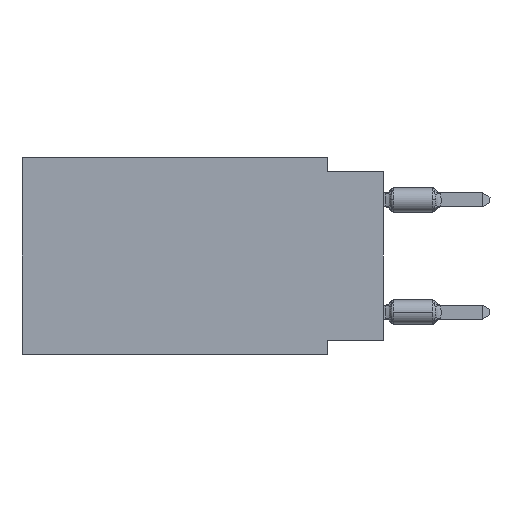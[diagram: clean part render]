
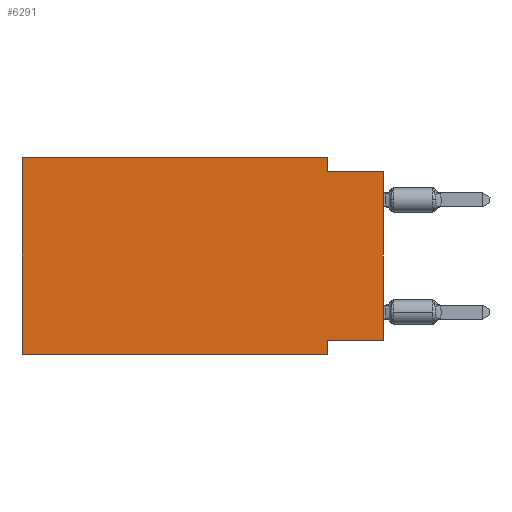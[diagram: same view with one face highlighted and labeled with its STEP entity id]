
A CAD part, left-side view. The second image highlights one B-rep face of the part: STEP entity #6291.
In plain terms, the highlighted planar face has unit normal (-1, 0, 0).
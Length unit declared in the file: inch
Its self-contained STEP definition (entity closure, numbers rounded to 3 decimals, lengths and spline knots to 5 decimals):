
#45 = LINE ( 'NONE', #5375, #10427 ) ;
#446 = CARTESIAN_POINT ( 'NONE',  ( 0., 0., -0.025 ) ) ;
#465 = VERTEX_POINT ( 'NONE', #10690 ) ;
#578 = EDGE_CURVE ( 'NONE', #5020, #465, #1015, .T. ) ;
#708 = VECTOR ( 'NONE', #12342, 39.37008 ) ;
#867 = CARTESIAN_POINT ( 'NONE',  ( 0., 0.645, 0. ) ) ;
#999 = ORIENTED_EDGE ( 'NONE', *, *, #6677, .F. ) ;
#1015 = LINE ( 'NONE', #8559, #12239 ) ;
#1303 = DIRECTION ( 'NONE',  ( 0., -1., 0. ) ) ;
#1345 = VERTEX_POINT ( 'NONE', #13321 ) ;
#1365 = VERTEX_POINT ( 'NONE', #867 ) ;
#1923 = EDGE_CURVE ( 'NONE', #1345, #16106, #2112, .T. ) ;
#1957 = LINE ( 'NONE', #7144, #708 ) ;
#2112 = LINE ( 'NONE', #8470, #4435 ) ;
#2314 = CARTESIAN_POINT ( 'NONE',  ( 0., 0.645, -0.35 ) ) ;
#3099 = VECTOR ( 'NONE', #15239, 39.37008 ) ;
#3431 = ORIENTED_EDGE ( 'NONE', *, *, #15196, .T. ) ;
#4435 = VECTOR ( 'NONE', #7371, 39.37008 ) ;
#4548 = EDGE_CURVE ( 'NONE', #10278, #1345, #4813, .T. ) ;
#4651 = CARTESIAN_POINT ( 'NONE',  ( 0., 0., -0.325 ) ) ;
#4769 = ORIENTED_EDGE ( 'NONE', *, *, #1923, .F. ) ;
#4813 = LINE ( 'NONE', #4651, #7572 ) ;
#5020 = VERTEX_POINT ( 'NONE', #15263 ) ;
#5375 = CARTESIAN_POINT ( 'NONE',  ( 0., 0.645, -0.35 ) ) ;
#5572 = DIRECTION ( 'NONE',  ( 1., 0., 0. ) ) ;
#5813 = PLANE ( 'NONE',  #16420 ) ;
#6208 = LINE ( 'NONE', #16662, #3099 ) ;
#6236 = ORIENTED_EDGE ( 'NONE', *, *, #12957, .F. ) ;
#6291 = ADVANCED_FACE ( 'NONE', ( #8270 ), #5813, .F. ) ;
#6677 = EDGE_CURVE ( 'NONE', #465, #10074, #1957, .T. ) ;
#7144 = CARTESIAN_POINT ( 'NONE',  ( 0., 0., -0.025 ) ) ;
#7352 = DIRECTION ( 'NONE',  ( 0., 1., 0. ) ) ;
#7371 = DIRECTION ( 'NONE',  ( 0., 0., -1. ) ) ;
#7572 = VECTOR ( 'NONE', #7352, 39.37008 ) ;
#7975 = ORIENTED_EDGE ( 'NONE', *, *, #4548, .F. ) ;
#8068 = EDGE_LOOP ( 'NONE', ( #3431, #999, #8498, #12904, #6236, #13268, #4769, #7975 ) ) ;
#8270 = FACE_OUTER_BOUND ( 'NONE', #8068, .T. ) ;
#8356 = DIRECTION ( 'NONE',  ( 0., 0., -1. ) ) ;
#8470 = CARTESIAN_POINT ( 'NONE',  ( 0., 0.1, -0.35 ) ) ;
#8498 = ORIENTED_EDGE ( 'NONE', *, *, #578, .F. ) ;
#8559 = CARTESIAN_POINT ( 'NONE',  ( 0., 0.1, 0. ) ) ;
#8575 = VECTOR ( 'NONE', #11095, 39.37008 ) ;
#9460 = CARTESIAN_POINT ( 'NONE',  ( 0., 0.645, 0. ) ) ;
#9985 = CARTESIAN_POINT ( 'NONE',  ( 0., 0.1, -0.35 ) ) ;
#10016 = DIRECTION ( 'NONE',  ( 0., 0., -1. ) ) ;
#10074 = VERTEX_POINT ( 'NONE', #446 ) ;
#10131 = CARTESIAN_POINT ( 'NONE',  ( 0., 0., -0.325 ) ) ;
#10278 = VERTEX_POINT ( 'NONE', #10131 ) ;
#10427 = VECTOR ( 'NONE', #1303, 39.37008 ) ;
#10690 = CARTESIAN_POINT ( 'NONE',  ( 0., 0.1, -0.025 ) ) ;
#10952 = VECTOR ( 'NONE', #15120, 39.37008 ) ;
#11095 = DIRECTION ( 'NONE',  ( 0., 0., 1. ) ) ;
#11168 = LINE ( 'NONE', #13772, #10952 ) ;
#11470 = VERTEX_POINT ( 'NONE', #2314 ) ;
#12239 = VECTOR ( 'NONE', #10016, 39.37008 ) ;
#12251 = EDGE_CURVE ( 'NONE', #1365, #5020, #11168, .T. ) ;
#12342 = DIRECTION ( 'NONE',  ( 0., -1., 0. ) ) ;
#12904 = ORIENTED_EDGE ( 'NONE', *, *, #12251, .F. ) ;
#12957 = EDGE_CURVE ( 'NONE', #11470, #1365, #6208, .T. ) ;
#13268 = ORIENTED_EDGE ( 'NONE', *, *, #16255, .T. ) ;
#13321 = CARTESIAN_POINT ( 'NONE',  ( 0., 0.1, -0.325 ) ) ;
#13772 = CARTESIAN_POINT ( 'NONE',  ( 0., 0.645, 0. ) ) ;
#15120 = DIRECTION ( 'NONE',  ( 0., -1., 0. ) ) ;
#15196 = EDGE_CURVE ( 'NONE', #10278, #10074, #16301, .T. ) ;
#15239 = DIRECTION ( 'NONE',  ( 0., 0., 1. ) ) ;
#15263 = CARTESIAN_POINT ( 'NONE',  ( 0., 0.1, 0. ) ) ;
#16061 = CARTESIAN_POINT ( 'NONE',  ( 0., 0., 0. ) ) ;
#16106 = VERTEX_POINT ( 'NONE', #9985 ) ;
#16255 = EDGE_CURVE ( 'NONE', #11470, #16106, #45, .T. ) ;
#16301 = LINE ( 'NONE', #16061, #8575 ) ;
#16420 = AXIS2_PLACEMENT_3D ( 'NONE', #9460, #5572, #8356 ) ;
#16662 = CARTESIAN_POINT ( 'NONE',  ( 0., 0.645, 0. ) ) ;
